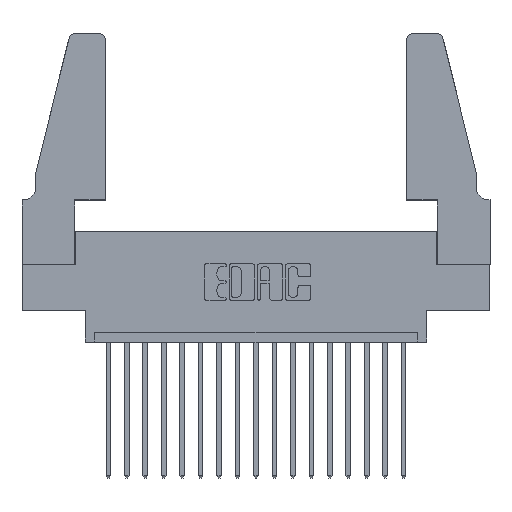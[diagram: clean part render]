
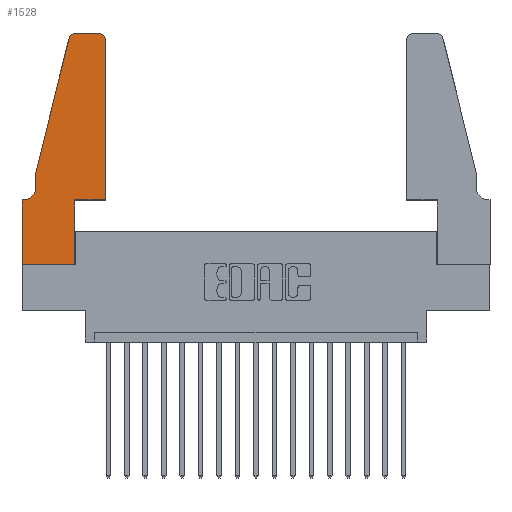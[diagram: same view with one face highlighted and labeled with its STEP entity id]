
A CAD part, top view. The second image highlights one B-rep face of the part: STEP entity #1528.
In plain terms, the highlighted planar face has unit normal (0, 0, 1).
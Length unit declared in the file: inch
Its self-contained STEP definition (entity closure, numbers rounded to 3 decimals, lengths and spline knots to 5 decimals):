
#351 = ORIENTED_EDGE ( 'NONE', *, *, #5881, .T. ) ;
#473 = ORIENTED_EDGE ( 'NONE', *, *, #15301, .T. ) ;
#477 = CIRCLE ( 'NONE', #12100, 0.07 ) ;
#595 = LINE ( 'NONE', #9655, #7681 ) ;
#682 = VECTOR ( 'NONE', #10731, 39.37008 ) ;
#697 = DIRECTION ( 'NONE',  ( 1., 0., 0. ) ) ;
#775 = DIRECTION ( 'NONE',  ( 0., -1., 0. ) ) ;
#1075 = ORIENTED_EDGE ( 'NONE', *, *, #18233, .T. ) ;
#1078 = DIRECTION ( 'NONE',  ( 0., 1., 0. ) ) ;
#1214 = VECTOR ( 'NONE', #775, 39.37008 ) ;
#1319 = VECTOR ( 'NONE', #17659, 39.37008 ) ;
#1528 = ADVANCED_FACE ( 'NONE', ( #14756 ), #6527, .T. ) ;
#1546 = LINE ( 'NONE', #17532, #1319 ) ;
#1655 = VECTOR ( 'NONE', #7407, 39.37008 ) ;
#2083 = CARTESIAN_POINT ( 'NONE',  ( 0., 0.35, 0.37 ) ) ;
#2470 = VERTEX_POINT ( 'NONE', #2083 ) ;
#2574 = DIRECTION ( 'NONE',  ( 0., 0., 1. ) ) ;
#2721 = VECTOR ( 'NONE', #7494, 39.37008 ) ;
#3044 = CARTESIAN_POINT ( 'NONE',  ( 0.2865, 0.35, 0.37 ) ) ;
#3058 = EDGE_CURVE ( 'NONE', #5219, #10208, #3875, .T. ) ;
#3149 = LINE ( 'NONE', #11886, #2721 ) ;
#3641 = DIRECTION ( 'NONE',  ( 0., 0., -1. ) ) ;
#3875 = LINE ( 'NONE', #18336, #5223 ) ;
#4226 = CARTESIAN_POINT ( 'NONE',  ( 0.25487, 1.22718, 0.37 ) ) ;
#4291 = DIRECTION ( 'NONE',  ( -0.239, -0.971, 0. ) ) ;
#4461 = CARTESIAN_POINT ( 'NONE',  ( 0.4505, 0.35, 0.37 ) ) ;
#4466 = LINE ( 'NONE', #5009, #682 ) ;
#5009 = CARTESIAN_POINT ( 'NONE',  ( 0.4505, 0.35, 0.37 ) ) ;
#5122 = DIRECTION ( 'NONE',  ( 0., 0., 1. ) ) ;
#5219 = VERTEX_POINT ( 'NONE', #4226 ) ;
#5223 = VECTOR ( 'NONE', #4291, 39.37008 ) ;
#5450 = LINE ( 'NONE', #11797, #1655 ) ;
#5565 = ORIENTED_EDGE ( 'NONE', *, *, #9571, .T. ) ;
#5856 = AXIS2_PLACEMENT_3D ( 'NONE', #18378, #2574, #13965 ) ;
#5881 = EDGE_CURVE ( 'NONE', #13579, #7302, #1546, .T. ) ;
#5893 = CIRCLE ( 'NONE', #6685, 0.03 ) ;
#5946 = CARTESIAN_POINT ( 'NONE',  ( 0.4505, 1.22, 0.37 ) ) ;
#6242 = EDGE_CURVE ( 'NONE', #7319, #5219, #16697, .T. ) ;
#6527 = PLANE ( 'NONE',  #9522 ) ;
#6544 = CARTESIAN_POINT ( 'NONE',  ( 0.0055, 0.42, 0.37 ) ) ;
#6685 = AXIS2_PLACEMENT_3D ( 'NONE', #17601, #7585, #697 ) ;
#6740 = CARTESIAN_POINT ( 'NONE',  ( 0., 0., 0.37 ) ) ;
#7302 = VERTEX_POINT ( 'NONE', #3044 ) ;
#7303 = LINE ( 'NONE', #16096, #12911 ) ;
#7319 = VERTEX_POINT ( 'NONE', #15545 ) ;
#7380 = LINE ( 'NONE', #11417, #8505 ) ;
#7407 = DIRECTION ( 'NONE',  ( 1., 0., 0. ) ) ;
#7494 = DIRECTION ( 'NONE',  ( -1., 0., 0. ) ) ;
#7585 = DIRECTION ( 'NONE',  ( 0., 0., 1. ) ) ;
#7681 = VECTOR ( 'NONE', #1078, 39.37008 ) ;
#7960 = DIRECTION ( 'NONE',  ( 1., 0., 0. ) ) ;
#8505 = VECTOR ( 'NONE', #8671, 39.37008 ) ;
#8671 = DIRECTION ( 'NONE',  ( 0., -1., 0. ) ) ;
#9102 = ORIENTED_EDGE ( 'NONE', *, *, #17187, .T. ) ;
#9418 = VERTEX_POINT ( 'NONE', #11604 ) ;
#9492 = ORIENTED_EDGE ( 'NONE', *, *, #12999, .T. ) ;
#9517 = EDGE_CURVE ( 'NONE', #14589, #13579, #5450, .T. ) ;
#9522 = AXIS2_PLACEMENT_3D ( 'NONE', #16534, #5122, #7960 ) ;
#9571 = EDGE_CURVE ( 'NONE', #10208, #9418, #15039, .T. ) ;
#9655 = CARTESIAN_POINT ( 'NONE',  ( 0.4505, 0.35, 0.37 ) ) ;
#9660 = ORIENTED_EDGE ( 'NONE', *, *, #3058, .T. ) ;
#10208 = VERTEX_POINT ( 'NONE', #10305 ) ;
#10305 = CARTESIAN_POINT ( 'NONE',  ( 0.0755, 0.5, 0.37 ) ) ;
#10382 = VERTEX_POINT ( 'NONE', #11862 ) ;
#10668 = ORIENTED_EDGE ( 'NONE', *, *, #9517, .T. ) ;
#10731 = DIRECTION ( 'NONE',  ( 1., 0., 0. ) ) ;
#10790 = ORIENTED_EDGE ( 'NONE', *, *, #17792, .T. ) ;
#11349 = ORIENTED_EDGE ( 'NONE', *, *, #6242, .T. ) ;
#11417 = CARTESIAN_POINT ( 'NONE',  ( 0., 0., 0.37 ) ) ;
#11604 = CARTESIAN_POINT ( 'NONE',  ( 0.0755, 0.42, 0.37 ) ) ;
#11772 = VERTEX_POINT ( 'NONE', #4461 ) ;
#11780 = EDGE_LOOP ( 'NONE', ( #9492, #11349, #9660, #5565, #1075, #10790, #9102, #10668, #351, #13190, #473, #14010 ) ) ;
#11797 = CARTESIAN_POINT ( 'NONE',  ( 0., 0., 0.37 ) ) ;
#11862 = CARTESIAN_POINT ( 'NONE',  ( 0.4205, 1.25, 0.37 ) ) ;
#11886 = CARTESIAN_POINT ( 'NONE',  ( 0.0755, 0.35, 0.37 ) ) ;
#12100 = AXIS2_PLACEMENT_3D ( 'NONE', #6544, #3641, #16613 ) ;
#12911 = VECTOR ( 'NONE', #13208, 39.37008 ) ;
#12999 = EDGE_CURVE ( 'NONE', #10382, #7319, #7303, .T. ) ;
#13117 = CARTESIAN_POINT ( 'NONE',  ( 0.0055, 0.35, 0.37 ) ) ;
#13190 = ORIENTED_EDGE ( 'NONE', *, *, #18238, .T. ) ;
#13208 = DIRECTION ( 'NONE',  ( -1., 0., 0. ) ) ;
#13316 = VERTEX_POINT ( 'NONE', #5946 ) ;
#13451 = VERTEX_POINT ( 'NONE', #13117 ) ;
#13579 = VERTEX_POINT ( 'NONE', #16703 ) ;
#13965 = DIRECTION ( 'NONE',  ( 1., 0., 0. ) ) ;
#14010 = ORIENTED_EDGE ( 'NONE', *, *, #15599, .T. ) ;
#14589 = VERTEX_POINT ( 'NONE', #6740 ) ;
#14756 = FACE_OUTER_BOUND ( 'NONE', #11780, .T. ) ;
#15039 = LINE ( 'NONE', #16245, #1214 ) ;
#15301 = EDGE_CURVE ( 'NONE', #11772, #13316, #595, .T. ) ;
#15545 = CARTESIAN_POINT ( 'NONE',  ( 0.284, 1.25, 0.37 ) ) ;
#15599 = EDGE_CURVE ( 'NONE', #13316, #10382, #5893, .T. ) ;
#16096 = CARTESIAN_POINT ( 'NONE',  ( 0.2605, 1.25, 0.37 ) ) ;
#16245 = CARTESIAN_POINT ( 'NONE',  ( 0.0755, 0.5, 0.37 ) ) ;
#16534 = CARTESIAN_POINT ( 'NONE',  ( 0., 0.35, 0.37 ) ) ;
#16613 = DIRECTION ( 'NONE',  ( -1., 0., 0. ) ) ;
#16697 = CIRCLE ( 'NONE', #5856, 0.03 ) ;
#16703 = CARTESIAN_POINT ( 'NONE',  ( 0.2865, 0., 0.37 ) ) ;
#17187 = EDGE_CURVE ( 'NONE', #2470, #14589, #7380, .T. ) ;
#17532 = CARTESIAN_POINT ( 'NONE',  ( 0.2865, 0.35, 0.37 ) ) ;
#17601 = CARTESIAN_POINT ( 'NONE',  ( 0.4205, 1.22, 0.37 ) ) ;
#17659 = DIRECTION ( 'NONE',  ( 0., 1., 0. ) ) ;
#17792 = EDGE_CURVE ( 'NONE', #13451, #2470, #3149, .T. ) ;
#18233 = EDGE_CURVE ( 'NONE', #9418, #13451, #477, .T. ) ;
#18238 = EDGE_CURVE ( 'NONE', #7302, #11772, #4466, .T. ) ;
#18336 = CARTESIAN_POINT ( 'NONE',  ( 0.0755, 0.5, 0.37 ) ) ;
#18378 = CARTESIAN_POINT ( 'NONE',  ( 0.284, 1.22, 0.37 ) ) ;
